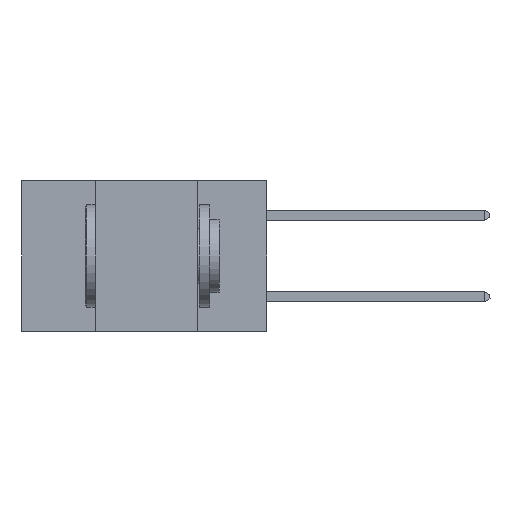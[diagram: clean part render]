
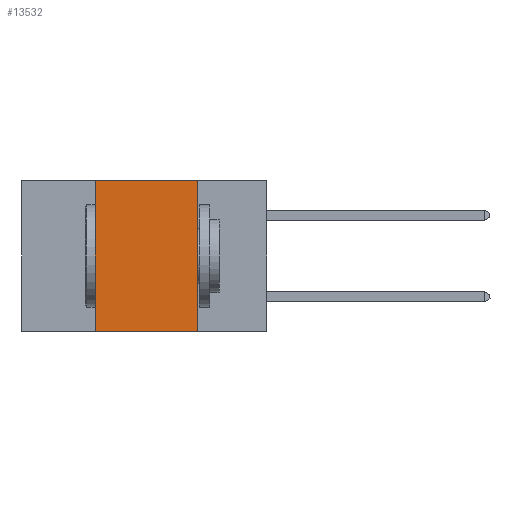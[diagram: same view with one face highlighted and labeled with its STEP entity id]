
A CAD part, left-side view. The second image highlights one B-rep face of the part: STEP entity #13532.
In plain terms, the highlighted planar face has unit normal (-1, 0, 0).
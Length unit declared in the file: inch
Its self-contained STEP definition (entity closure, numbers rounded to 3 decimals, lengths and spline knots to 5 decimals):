
#639 = CARTESIAN_POINT ( 'NONE',  ( 0., 0.6, -0.37 ) ) ;
#1142 = VERTEX_POINT ( 'NONE', #3421 ) ;
#1627 = CARTESIAN_POINT ( 'NONE',  ( 0., 0.42, 0. ) ) ;
#2502 = LINE ( 'NONE', #1627, #2975 ) ;
#2975 = VECTOR ( 'NONE', #10280, 39.37008 ) ;
#3421 = CARTESIAN_POINT ( 'NONE',  ( 0., 0.42, 0. ) ) ;
#4078 = DIRECTION ( 'NONE',  ( 1., 0., 0. ) ) ;
#4868 = LINE ( 'NONE', #639, #8635 ) ;
#4898 = EDGE_CURVE ( 'NONE', #1142, #14034, #7063, .T. ) ;
#6336 = EDGE_CURVE ( 'NONE', #13831, #1142, #2502, .T. ) ;
#6664 = ORIENTED_EDGE ( 'NONE', *, *, #9164, .F. ) ;
#6684 = AXIS2_PLACEMENT_3D ( 'NONE', #12453, #4078, #13808 ) ;
#6886 = PLANE ( 'NONE',  #6684 ) ;
#7063 = LINE ( 'NONE', #9986, #17510 ) ;
#7172 = DIRECTION ( 'NONE',  ( 0., -1., 0. ) ) ;
#7781 = DIRECTION ( 'NONE',  ( 0., 0., -1. ) ) ;
#7983 = LINE ( 'NONE', #15965, #14828 ) ;
#8635 = VECTOR ( 'NONE', #9376, 39.37008 ) ;
#9164 = EDGE_CURVE ( 'NONE', #14034, #10515, #7983, .T. ) ;
#9376 = DIRECTION ( 'NONE',  ( 0., -1., 0. ) ) ;
#9653 = CARTESIAN_POINT ( 'NONE',  ( 0., 0.17, -0.37 ) ) ;
#9986 = CARTESIAN_POINT ( 'NONE',  ( 0., 0.6, 0. ) ) ;
#10280 = DIRECTION ( 'NONE',  ( 0., 0., 1. ) ) ;
#10515 = VERTEX_POINT ( 'NONE', #9653 ) ;
#12399 = FACE_OUTER_BOUND ( 'NONE', #14486, .T. ) ;
#12453 = CARTESIAN_POINT ( 'NONE',  ( 0., 0.6, 0. ) ) ;
#13532 = ADVANCED_FACE ( 'NONE', ( #12399 ), #6886, .F. ) ;
#13808 = DIRECTION ( 'NONE',  ( 0., 0., -1. ) ) ;
#13831 = VERTEX_POINT ( 'NONE', #15767 ) ;
#13985 = ORIENTED_EDGE ( 'NONE', *, *, #4898, .F. ) ;
#14034 = VERTEX_POINT ( 'NONE', #17537 ) ;
#14396 = ORIENTED_EDGE ( 'NONE', *, *, #6336, .F. ) ;
#14486 = EDGE_LOOP ( 'NONE', ( #6664, #13985, #14396, #17961 ) ) ;
#14828 = VECTOR ( 'NONE', #7781, 39.37008 ) ;
#15767 = CARTESIAN_POINT ( 'NONE',  ( 0., 0.42, -0.37 ) ) ;
#15965 = CARTESIAN_POINT ( 'NONE',  ( 0., 0.17, 0. ) ) ;
#17510 = VECTOR ( 'NONE', #7172, 39.37008 ) ;
#17537 = CARTESIAN_POINT ( 'NONE',  ( 0., 0.17, 0. ) ) ;
#17636 = EDGE_CURVE ( 'NONE', #13831, #10515, #4868, .T. ) ;
#17961 = ORIENTED_EDGE ( 'NONE', *, *, #17636, .T. ) ;
